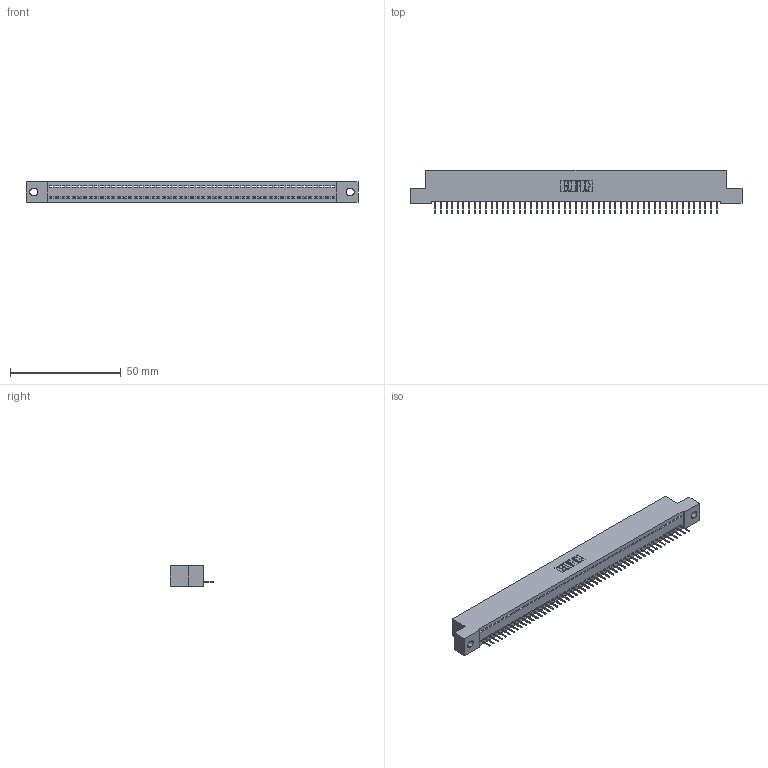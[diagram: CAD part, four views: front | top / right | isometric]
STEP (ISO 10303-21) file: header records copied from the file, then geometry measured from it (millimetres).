
FILE_DESCRIPTION (( 'STEP AP203' ), '1' );
FILE_NAME ('392-051-524-102.STEP', '2018-08-17T03:36:12', ( '' ), ( '' ), 'SwSTEP 2.0', 'SolidWorks 2016', '' );
FILE_SCHEMA (( 'CONFIG_CONTROL_DESIGN' ));
Length unit declared in the file: inch
Products named in the file (3): 345-292-001_345-293-124; 392-051-524-102; 342 Part_.128 Slot
Assembly tree (52 placements, depth 2):
  392-051-524-102
    342 Part_.128 Slot
    345-292-001_345-293-124  x51
Bounding box: 149.86 x 19.69 x 9.4 mm (x, y, z)
Volume: 12919.3 mm3; surface area: 18273.3 mm2
Topology: 52 solids, 52 shells, 3276 faces, 9491 edges, 6122 vertices
Faces by surface type: plane 2518, cylinder 758
Entity records: 30091 total; most frequent: CARTESIAN_POINT 5195, ORIENTED_EDGE 5182, DIRECTION 4365, EDGE_CURVE 2591, LINE 2467, VECTOR 2467, VERTEX_POINT 1722, AXIS2_PLACEMENT_3D 949
